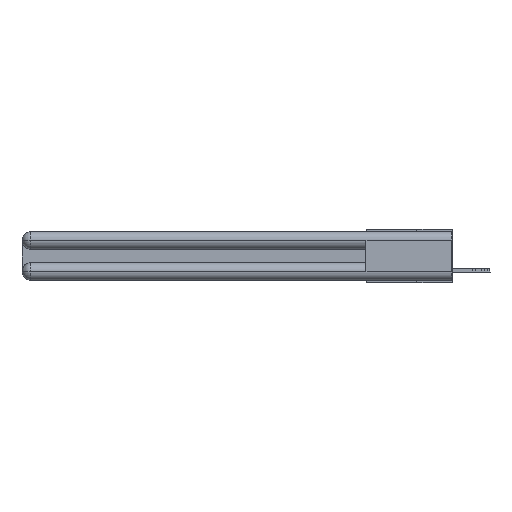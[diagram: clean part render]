
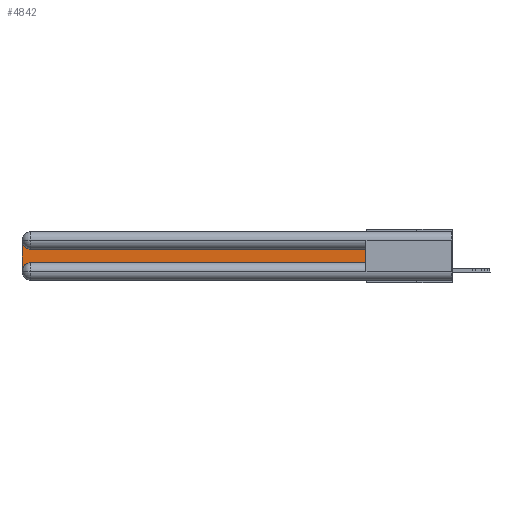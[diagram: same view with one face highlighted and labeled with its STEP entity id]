
A CAD part, left-side view. The second image highlights one B-rep face of the part: STEP entity #4842.
In plain terms, the highlighted planar face has unit normal (-1, 0, 0).
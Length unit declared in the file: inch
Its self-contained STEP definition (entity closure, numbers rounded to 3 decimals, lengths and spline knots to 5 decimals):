
#1281 = CARTESIAN_POINT ( 'NONE',  ( 0.075, 0.6, -0.1225 ) ) ;
#1373 = VECTOR ( 'NONE', #14578, 39.37008 ) ;
#1948 = EDGE_CURVE ( 'NONE', #5255, #16150, #12689, .T. ) ;
#2043 = ORIENTED_EDGE ( 'NONE', *, *, #1948, .T. ) ;
#2498 = CARTESIAN_POINT ( 'NONE',  ( 0.075, 2.94, -0.0625 ) ) ;
#2518 = CARTESIAN_POINT ( 'NONE',  ( 0.075, 2.94, -0.2175 ) ) ;
#2796 = EDGE_CURVE ( 'NONE', #15180, #27932, #31170, .T. ) ;
#2955 = DIRECTION ( 'NONE',  ( 1., 0., 0. ) ) ;
#3030 = EDGE_CURVE ( 'NONE', #16150, #4278, #24357, .T. ) ;
#3164 = PLANE ( 'NONE',  #20069 ) ;
#3590 = ORIENTED_EDGE ( 'NONE', *, *, #2796, .T. ) ;
#4278 = VERTEX_POINT ( 'NONE', #5020 ) ;
#4364 = VECTOR ( 'NONE', #24618, 39.37008 ) ;
#4842 = ADVANCED_FACE ( 'NONE', ( #15655 ), #3164, .F. ) ;
#5020 = CARTESIAN_POINT ( 'NONE',  ( 0.075, 3., -0.0625 ) ) ;
#5255 = VERTEX_POINT ( 'NONE', #1281 ) ;
#5295 = CARTESIAN_POINT ( 'NONE',  ( 0.075, 0.6, -0.2175 ) ) ;
#5907 = EDGE_CURVE ( 'NONE', #18076, #15180, #22379, .T. ) ;
#7409 = AXIS2_PLACEMENT_3D ( 'NONE', #12547, #29451, #14948 ) ;
#7925 = CARTESIAN_POINT ( 'NONE',  ( 0.075, 0.6, -0.1225 ) ) ;
#8060 = ORIENTED_EDGE ( 'NONE', *, *, #3030, .T. ) ;
#8230 = VECTOR ( 'NONE', #13620, 39.37008 ) ;
#8781 = CARTESIAN_POINT ( 'NONE',  ( 0.075, 0.6, -0.2175 ) ) ;
#9003 = ORIENTED_EDGE ( 'NONE', *, *, #12564, .T. ) ;
#9964 = AXIS2_PLACEMENT_3D ( 'NONE', #2498, #24260, #29104 ) ;
#10439 = CARTESIAN_POINT ( 'NONE',  ( 0.075, 3., -0.1225 ) ) ;
#11617 = CARTESIAN_POINT ( 'NONE',  ( 0.075, 2.94, -0.1225 ) ) ;
#12547 = CARTESIAN_POINT ( 'NONE',  ( 0.075, 2.94, -0.2775 ) ) ;
#12564 = EDGE_CURVE ( 'NONE', #4278, #18076, #18721, .T. ) ;
#12627 = LINE ( 'NONE', #5295, #4364 ) ;
#12689 = LINE ( 'NONE', #7925, #8230 ) ;
#13066 = CARTESIAN_POINT ( 'NONE',  ( 0.075, 0.6, -0.2175 ) ) ;
#13410 = EDGE_CURVE ( 'NONE', #27932, #5255, #12627, .T. ) ;
#13620 = DIRECTION ( 'NONE',  ( 0., 1., 0. ) ) ;
#14578 = DIRECTION ( 'NONE',  ( 0., 0., -1. ) ) ;
#14948 = DIRECTION ( 'NONE',  ( 0., 0., -1. ) ) ;
#15069 = DIRECTION ( 'NONE',  ( 0., 0., -1. ) ) ;
#15180 = VERTEX_POINT ( 'NONE', #2518 ) ;
#15284 = EDGE_LOOP ( 'NONE', ( #2043, #8060, #9003, #30691, #3590, #17474 ) ) ;
#15655 = FACE_OUTER_BOUND ( 'NONE', #15284, .T. ) ;
#16150 = VERTEX_POINT ( 'NONE', #11617 ) ;
#17474 = ORIENTED_EDGE ( 'NONE', *, *, #13410, .T. ) ;
#18076 = VERTEX_POINT ( 'NONE', #25607 ) ;
#18721 = LINE ( 'NONE', #28885, #1373 ) ;
#20069 = AXIS2_PLACEMENT_3D ( 'NONE', #10439, #2955, #15069 ) ;
#20549 = VECTOR ( 'NONE', #29982, 39.37008 ) ;
#22379 = CIRCLE ( 'NONE', #7409, 0.06 ) ;
#24260 = DIRECTION ( 'NONE',  ( 1., 0., 0. ) ) ;
#24357 = CIRCLE ( 'NONE', #9964, 0.06 ) ;
#24618 = DIRECTION ( 'NONE',  ( 0., 0., 1. ) ) ;
#25607 = CARTESIAN_POINT ( 'NONE',  ( 0.075, 3., -0.2775 ) ) ;
#27932 = VERTEX_POINT ( 'NONE', #8781 ) ;
#28885 = CARTESIAN_POINT ( 'NONE',  ( 0.075, 3., -0.2175 ) ) ;
#29104 = DIRECTION ( 'NONE',  ( 0., 0., -1. ) ) ;
#29451 = DIRECTION ( 'NONE',  ( 1., 0., 0. ) ) ;
#29982 = DIRECTION ( 'NONE',  ( 0., -1., 0. ) ) ;
#30691 = ORIENTED_EDGE ( 'NONE', *, *, #5907, .T. ) ;
#31170 = LINE ( 'NONE', #13066, #20549 ) ;
